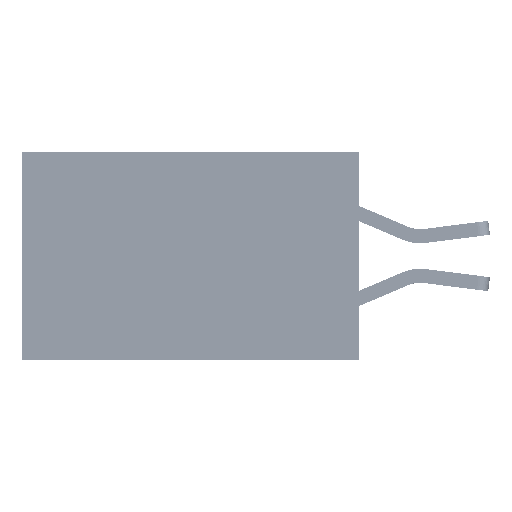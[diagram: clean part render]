
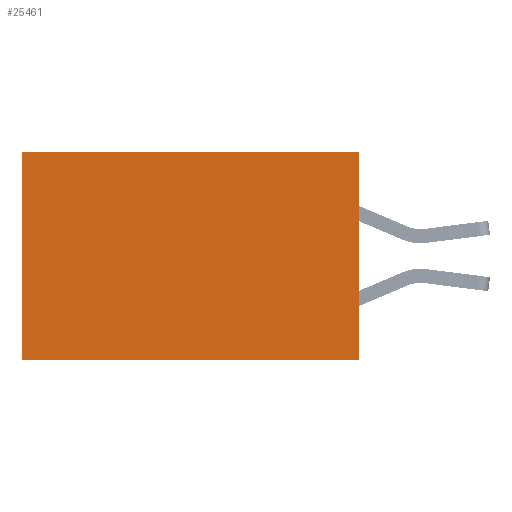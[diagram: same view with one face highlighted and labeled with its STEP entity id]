
A CAD part, left-side view. The second image highlights one B-rep face of the part: STEP entity #25461.
In plain terms, the highlighted planar face has unit normal (-1, 0, 0).
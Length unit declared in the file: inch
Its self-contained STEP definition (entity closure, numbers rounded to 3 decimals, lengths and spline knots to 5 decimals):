
#1966 = EDGE_LOOP ( 'NONE', ( #16645, #22528, #14482, #8351 ) ) ;
#3711 = VECTOR ( 'NONE', #20027, 39.37008 ) ;
#4143 = DIRECTION ( 'NONE',  ( 0., 0., -1. ) ) ;
#5561 = EDGE_CURVE ( 'NONE', #15343, #17671, #11142, .T. ) ;
#6228 = DIRECTION ( 'NONE',  ( 0., 0., -1. ) ) ;
#8351 = ORIENTED_EDGE ( 'NONE', *, *, #17475, .T. ) ;
#9325 = VECTOR ( 'NONE', #4143, 39.37008 ) ;
#11000 = CARTESIAN_POINT ( 'NONE',  ( 0.2875, 0., 0. ) ) ;
#11142 = LINE ( 'NONE', #20280, #3711 ) ;
#11948 = LINE ( 'NONE', #32069, #9325 ) ;
#12784 = EDGE_CURVE ( 'NONE', #17042, #17671, #11948, .T. ) ;
#13610 = CARTESIAN_POINT ( 'NONE',  ( 0.2875, 0., -0.37 ) ) ;
#14133 = LINE ( 'NONE', #36245, #21186 ) ;
#14482 = ORIENTED_EDGE ( 'NONE', *, *, #31721, .F. ) ;
#14763 = FACE_OUTER_BOUND ( 'NONE', #1966, .T. ) ;
#14770 = CARTESIAN_POINT ( 'NONE',  ( 0.2875, 0., 0. ) ) ;
#15343 = VERTEX_POINT ( 'NONE', #13610 ) ;
#16299 = CARTESIAN_POINT ( 'NONE',  ( 0.2875, 0., 0. ) ) ;
#16645 = ORIENTED_EDGE ( 'NONE', *, *, #12784, .T. ) ;
#17042 = VERTEX_POINT ( 'NONE', #31751 ) ;
#17412 = VECTOR ( 'NONE', #19132, 39.37008 ) ;
#17475 = EDGE_CURVE ( 'NONE', #26646, #17042, #14133, .T. ) ;
#17671 = VERTEX_POINT ( 'NONE', #28167 ) ;
#19132 = DIRECTION ( 'NONE',  ( 0., 0., -1. ) ) ;
#20027 = DIRECTION ( 'NONE',  ( 0., 1., 0. ) ) ;
#20280 = CARTESIAN_POINT ( 'NONE',  ( 0.2875, 0., -0.37 ) ) ;
#21186 = VECTOR ( 'NONE', #30251, 39.37008 ) ;
#22528 = ORIENTED_EDGE ( 'NONE', *, *, #5561, .F. ) ;
#23036 = DIRECTION ( 'NONE',  ( 1., 0., 0. ) ) ;
#24897 = AXIS2_PLACEMENT_3D ( 'NONE', #11000, #23036, #6228 ) ;
#25461 = ADVANCED_FACE ( 'NONE', ( #14763 ), #30495, .F. ) ;
#26637 = LINE ( 'NONE', #16299, #17412 ) ;
#26646 = VERTEX_POINT ( 'NONE', #14770 ) ;
#28167 = CARTESIAN_POINT ( 'NONE',  ( 0.2875, 0.6, -0.37 ) ) ;
#30251 = DIRECTION ( 'NONE',  ( 0., 1., 0. ) ) ;
#30495 = PLANE ( 'NONE',  #24897 ) ;
#31721 = EDGE_CURVE ( 'NONE', #26646, #15343, #26637, .T. ) ;
#31751 = CARTESIAN_POINT ( 'NONE',  ( 0.2875, 0.6, 0. ) ) ;
#32069 = CARTESIAN_POINT ( 'NONE',  ( 0.2875, 0.6, 0. ) ) ;
#36245 = CARTESIAN_POINT ( 'NONE',  ( 0.2875, 0., 0. ) ) ;
